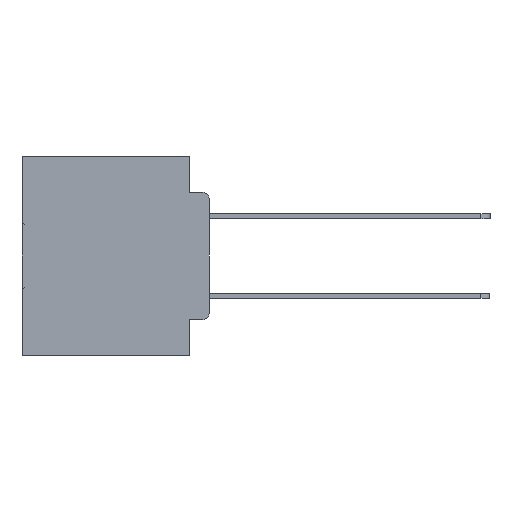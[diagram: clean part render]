
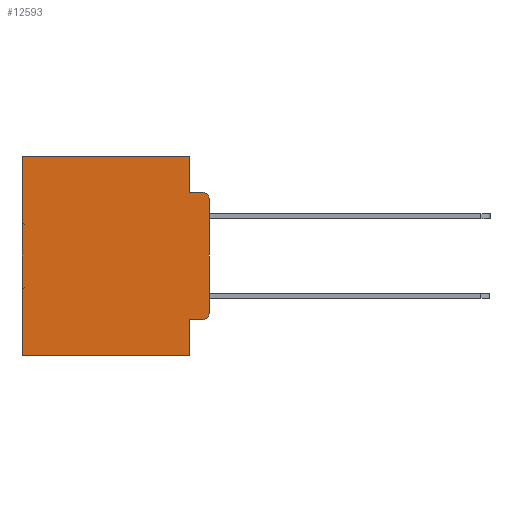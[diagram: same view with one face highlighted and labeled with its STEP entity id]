
A CAD part, left-side view. The second image highlights one B-rep face of the part: STEP entity #12593.
In plain terms, the highlighted planar face has unit normal (-1, 0, 0).
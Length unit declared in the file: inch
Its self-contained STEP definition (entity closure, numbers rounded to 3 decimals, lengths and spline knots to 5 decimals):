
#93 = VECTOR ( 'NONE', #27027, 39.37008 ) ;
#308 = EDGE_CURVE ( 'NONE', #1042, #16428, #23991, .T. ) ;
#659 = AXIS2_PLACEMENT_3D ( 'NONE', #1436, #17682, #1554 ) ;
#708 = EDGE_CURVE ( 'NONE', #16589, #32983, #30032, .T. ) ;
#878 = VECTOR ( 'NONE', #31893, 39.37008 ) ;
#1042 = VERTEX_POINT ( 'NONE', #17618 ) ;
#1436 = CARTESIAN_POINT ( 'NONE',  ( 0.298, 0., 0. ) ) ;
#1554 = DIRECTION ( 'NONE',  ( 0., 0., -1. ) ) ;
#2031 = CARTESIAN_POINT ( 'NONE',  ( 0.298, 0.473, 0. ) ) ;
#2147 = DIRECTION ( 'NONE',  ( 0., 1., 0. ) ) ;
#2603 = DIRECTION ( 'NONE',  ( -1., 0., 0. ) ) ;
#3168 = ORIENTED_EDGE ( 'NONE', *, *, #19161, .T. ) ;
#3354 = LINE ( 'NONE', #23327, #4208 ) ;
#3514 = CARTESIAN_POINT ( 'NONE',  ( 0.298, 0., 0. ) ) ;
#4208 = VECTOR ( 'NONE', #33634, 39.37008 ) ;
#4775 = VECTOR ( 'NONE', #24856, 39.37008 ) ;
#8793 = VERTEX_POINT ( 'NONE', #30328 ) ;
#8805 = CARTESIAN_POINT ( 'NONE',  ( 0.298, 0., -0.5 ) ) ;
#8938 = VECTOR ( 'NONE', #30791, 39.37008 ) ;
#8963 = VECTOR ( 'NONE', #2147, 39.37008 ) ;
#9840 = CARTESIAN_POINT ( 'NONE',  ( 0.298, 0.02, -0.3915 ) ) ;
#11795 = EDGE_CURVE ( 'NONE', #18252, #26429, #12320, .T. ) ;
#12222 = CARTESIAN_POINT ( 'NONE',  ( 0.298, 0.051, -0.4115 ) ) ;
#12320 = LINE ( 'NONE', #19191, #32460 ) ;
#12556 = DIRECTION ( 'NONE',  ( 0., 0., -1. ) ) ;
#12593 = ADVANCED_FACE ( 'NONE', ( #14769 ), #14984, .F. ) ;
#12864 = ORIENTED_EDGE ( 'NONE', *, *, #31614, .T. ) ;
#13736 = EDGE_CURVE ( 'NONE', #28926, #14734, #19009, .T. ) ;
#14141 = EDGE_LOOP ( 'NONE', ( #18261, #3168, #19919, #26915, #12864, #34202, #18712, #17511, #32632, #27769 ) ) ;
#14523 = CIRCLE ( 'NONE', #28918, 0.02 ) ;
#14734 = VERTEX_POINT ( 'NONE', #22308 ) ;
#14769 = FACE_OUTER_BOUND ( 'NONE', #14141, .T. ) ;
#14984 = PLANE ( 'NONE',  #659 ) ;
#16015 = AXIS2_PLACEMENT_3D ( 'NONE', #9840, #28343, #12556 ) ;
#16428 = VERTEX_POINT ( 'NONE', #21723 ) ;
#16553 = DIRECTION ( 'NONE',  ( 0., -1., 0. ) ) ;
#16589 = VERTEX_POINT ( 'NONE', #32650 ) ;
#17511 = ORIENTED_EDGE ( 'NONE', *, *, #22236, .F. ) ;
#17618 = CARTESIAN_POINT ( 'NONE',  ( 0.298, 0.051, 0. ) ) ;
#17682 = DIRECTION ( 'NONE',  ( 1., 0., 0. ) ) ;
#18252 = VERTEX_POINT ( 'NONE', #12222 ) ;
#18261 = ORIENTED_EDGE ( 'NONE', *, *, #13736, .F. ) ;
#18681 = CARTESIAN_POINT ( 'NONE',  ( 0.298, 0.02, -0.1085 ) ) ;
#18712 = ORIENTED_EDGE ( 'NONE', *, *, #708, .F. ) ;
#19009 = LINE ( 'NONE', #3514, #4775 ) ;
#19161 = EDGE_CURVE ( 'NONE', #28926, #8793, #14523, .T. ) ;
#19191 = CARTESIAN_POINT ( 'NONE',  ( 0.298, 0.051, -0.4115 ) ) ;
#19919 = ORIENTED_EDGE ( 'NONE', *, *, #28079, .F. ) ;
#21336 = DIRECTION ( 'NONE',  ( 0., 0., -1. ) ) ;
#21477 = CARTESIAN_POINT ( 'NONE',  ( 0.298, 0.473, 0. ) ) ;
#21611 = EDGE_CURVE ( 'NONE', #26429, #14734, #21795, .T. ) ;
#21723 = CARTESIAN_POINT ( 'NONE',  ( 0.298, 0.051, -0.0885 ) ) ;
#21795 = CIRCLE ( 'NONE', #16015, 0.02 ) ;
#22236 = EDGE_CURVE ( 'NONE', #18252, #16589, #3354, .T. ) ;
#22308 = CARTESIAN_POINT ( 'NONE',  ( 0.298, 0., -0.3915 ) ) ;
#23111 = LINE ( 'NONE', #26684, #878 ) ;
#23166 = LINE ( 'NONE', #33846, #8963 ) ;
#23327 = CARTESIAN_POINT ( 'NONE',  ( 0.298, 0.051, 0. ) ) ;
#23426 = CARTESIAN_POINT ( 'NONE',  ( 0.298, 0.473, -0.5 ) ) ;
#23991 = LINE ( 'NONE', #33954, #93 ) ;
#24856 = DIRECTION ( 'NONE',  ( 0., 0., -1. ) ) ;
#26429 = VERTEX_POINT ( 'NONE', #32663 ) ;
#26684 = CARTESIAN_POINT ( 'NONE',  ( 0.298, 0.051, -0.0885 ) ) ;
#26878 = VERTEX_POINT ( 'NONE', #21477 ) ;
#26915 = ORIENTED_EDGE ( 'NONE', *, *, #308, .F. ) ;
#27027 = DIRECTION ( 'NONE',  ( 0., 0., -1. ) ) ;
#27769 = ORIENTED_EDGE ( 'NONE', *, *, #21611, .T. ) ;
#28079 = EDGE_CURVE ( 'NONE', #16428, #8793, #23111, .T. ) ;
#28343 = DIRECTION ( 'NONE',  ( -1., 0., 0. ) ) ;
#28650 = DIRECTION ( 'NONE',  ( 0., 0., -1. ) ) ;
#28918 = AXIS2_PLACEMENT_3D ( 'NONE', #18681, #2603, #21336 ) ;
#28926 = VERTEX_POINT ( 'NONE', #32624 ) ;
#30032 = LINE ( 'NONE', #8805, #8938 ) ;
#30062 = VECTOR ( 'NONE', #28650, 39.37008 ) ;
#30328 = CARTESIAN_POINT ( 'NONE',  ( 0.298, 0.02, -0.0885 ) ) ;
#30791 = DIRECTION ( 'NONE',  ( 0., 1., 0. ) ) ;
#30885 = LINE ( 'NONE', #2031, #30062 ) ;
#31609 = EDGE_CURVE ( 'NONE', #26878, #32983, #30885, .T. ) ;
#31614 = EDGE_CURVE ( 'NONE', #1042, #26878, #23166, .T. ) ;
#31893 = DIRECTION ( 'NONE',  ( 0., -1., 0. ) ) ;
#32460 = VECTOR ( 'NONE', #16553, 39.37008 ) ;
#32624 = CARTESIAN_POINT ( 'NONE',  ( 0.298, 0., -0.1085 ) ) ;
#32632 = ORIENTED_EDGE ( 'NONE', *, *, #11795, .T. ) ;
#32650 = CARTESIAN_POINT ( 'NONE',  ( 0.298, 0.051, -0.5 ) ) ;
#32663 = CARTESIAN_POINT ( 'NONE',  ( 0.298, 0.02, -0.4115 ) ) ;
#32983 = VERTEX_POINT ( 'NONE', #23426 ) ;
#33634 = DIRECTION ( 'NONE',  ( 0., 0., -1. ) ) ;
#33846 = CARTESIAN_POINT ( 'NONE',  ( 0.298, 0., 0. ) ) ;
#33954 = CARTESIAN_POINT ( 'NONE',  ( 0.298, 0.051, 0. ) ) ;
#34202 = ORIENTED_EDGE ( 'NONE', *, *, #31609, .T. ) ;
